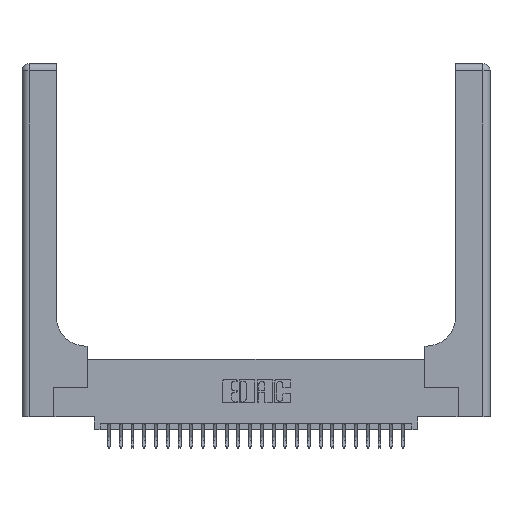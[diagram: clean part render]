
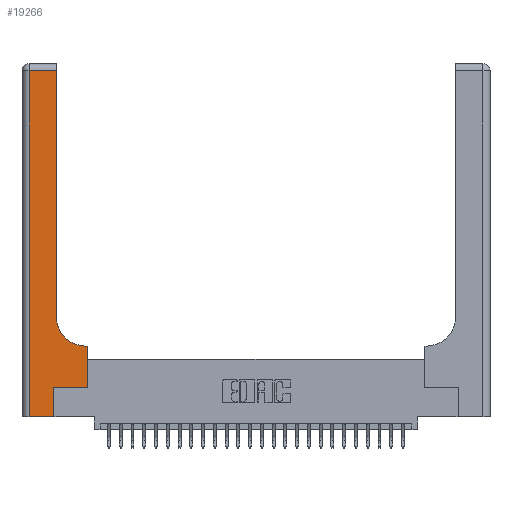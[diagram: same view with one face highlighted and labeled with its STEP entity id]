
A CAD part, top view. The second image highlights one B-rep face of the part: STEP entity #19266.
In plain terms, the highlighted planar face has unit normal (0, 0, 1).
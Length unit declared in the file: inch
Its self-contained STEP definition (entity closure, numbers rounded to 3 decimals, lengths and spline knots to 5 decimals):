
#473 = CARTESIAN_POINT ( 'NONE',  ( 0.2915, 2.94, 0.37 ) ) ;
#1381 = DIRECTION ( 'NONE',  ( 0., 1., 0. ) ) ;
#1568 = CARTESIAN_POINT ( 'NONE',  ( 0.5585, 0.25, 0.37 ) ) ;
#1997 = VERTEX_POINT ( 'NONE', #9951 ) ;
#2394 = FACE_OUTER_BOUND ( 'NONE', #5670, .T. ) ;
#3526 = ORIENTED_EDGE ( 'NONE', *, *, #18394, .T. ) ;
#3707 = CARTESIAN_POINT ( 'NONE',  ( 0.2915, 3., 0.37 ) ) ;
#3811 = DIRECTION ( 'NONE',  ( -1., 0., 0. ) ) ;
#3971 = DIRECTION ( 'NONE',  ( 0., 1., 0. ) ) ;
#4874 = DIRECTION ( 'NONE',  ( -1., 0., 0. ) ) ;
#4939 = CIRCLE ( 'NONE', #16758, 0.25 ) ;
#5670 = EDGE_LOOP ( 'NONE', ( #16331, #16443, #14378, #25839, #3526, #7637, #23231, #17557, #17245 ) ) ;
#6155 = LINE ( 'NONE', #1568, #26515 ) ;
#6334 = EDGE_CURVE ( 'NONE', #27411, #19929, #20702, .T. ) ;
#7045 = VERTEX_POINT ( 'NONE', #473 ) ;
#7300 = EDGE_CURVE ( 'NONE', #12934, #10145, #14510, .T. ) ;
#7441 = VECTOR ( 'NONE', #1381, 39.37008 ) ;
#7637 = ORIENTED_EDGE ( 'NONE', *, *, #22457, .T. ) ;
#8154 = CARTESIAN_POINT ( 'NONE',  ( 0., 2.94, 0.37 ) ) ;
#8355 = VECTOR ( 'NONE', #15981, 39.37008 ) ;
#8759 = CARTESIAN_POINT ( 'NONE',  ( 0.06, 3., 0.37 ) ) ;
#9126 = CARTESIAN_POINT ( 'NONE',  ( 0., 0., 0.37 ) ) ;
#9167 = DIRECTION ( 'NONE',  ( 0., 1., 0. ) ) ;
#9366 = CARTESIAN_POINT ( 'NONE',  ( 0.269, 0.25, 0.37 ) ) ;
#9592 = VECTOR ( 'NONE', #9167, 39.37008 ) ;
#9951 = CARTESIAN_POINT ( 'NONE',  ( 0.5585, 0.25, 0.37 ) ) ;
#10145 = VERTEX_POINT ( 'NONE', #27791 ) ;
#10206 = VERTEX_POINT ( 'NONE', #25548 ) ;
#11107 = CARTESIAN_POINT ( 'NONE',  ( 0., 3., 0.37 ) ) ;
#11243 = DIRECTION ( 'NONE',  ( 0., 0., -1. ) ) ;
#11430 = CARTESIAN_POINT ( 'NONE',  ( 0.2915, 0.6, 0.37 ) ) ;
#11555 = VECTOR ( 'NONE', #3811, 39.37008 ) ;
#12934 = VERTEX_POINT ( 'NONE', #14967 ) ;
#12981 = VERTEX_POINT ( 'NONE', #15341 ) ;
#13124 = DIRECTION ( 'NONE',  ( 0., -1., 0. ) ) ;
#13723 = CARTESIAN_POINT ( 'NONE',  ( 0.5415, 0.6, 0.37 ) ) ;
#14378 = ORIENTED_EDGE ( 'NONE', *, *, #7300, .T. ) ;
#14384 = CARTESIAN_POINT ( 'NONE',  ( 0.2915, 0.85, 0.37 ) ) ;
#14467 = EDGE_CURVE ( 'NONE', #10145, #10206, #18913, .T. ) ;
#14510 = LINE ( 'NONE', #8759, #19618 ) ;
#14879 = LINE ( 'NONE', #3707, #7441 ) ;
#14967 = CARTESIAN_POINT ( 'NONE',  ( 0.06, 2.94, 0.37 ) ) ;
#15284 = PLANE ( 'NONE',  #17898 ) ;
#15341 = CARTESIAN_POINT ( 'NONE',  ( 0.269, 0.25, 0.37 ) ) ;
#15981 = DIRECTION ( 'NONE',  ( 1., 0., 0. ) ) ;
#16331 = ORIENTED_EDGE ( 'NONE', *, *, #20767, .T. ) ;
#16443 = ORIENTED_EDGE ( 'NONE', *, *, #19646, .T. ) ;
#16758 = AXIS2_PLACEMENT_3D ( 'NONE', #26977, #11243, #26426 ) ;
#16892 = LINE ( 'NONE', #9366, #23323 ) ;
#17168 = EDGE_CURVE ( 'NONE', #19929, #25767, #4939, .T. ) ;
#17245 = ORIENTED_EDGE ( 'NONE', *, *, #17168, .T. ) ;
#17557 = ORIENTED_EDGE ( 'NONE', *, *, #6334, .T. ) ;
#17898 = AXIS2_PLACEMENT_3D ( 'NONE', #11107, #19869, #4874 ) ;
#18111 = CARTESIAN_POINT ( 'NONE',  ( 0.269, 0., 0.37 ) ) ;
#18394 = EDGE_CURVE ( 'NONE', #10206, #12981, #25899, .T. ) ;
#18913 = LINE ( 'NONE', #9126, #8355 ) ;
#19266 = ADVANCED_FACE ( 'NONE', ( #2394 ), #15284, .F. ) ;
#19618 = VECTOR ( 'NONE', #13124, 39.37008 ) ;
#19646 = EDGE_CURVE ( 'NONE', #7045, #12934, #23104, .T. ) ;
#19869 = DIRECTION ( 'NONE',  ( 0., 0., -1. ) ) ;
#19929 = VERTEX_POINT ( 'NONE', #13723 ) ;
#20702 = LINE ( 'NONE', #11430, #23734 ) ;
#20767 = EDGE_CURVE ( 'NONE', #25767, #7045, #14879, .T. ) ;
#20924 = CARTESIAN_POINT ( 'NONE',  ( 0.5585, 0.6, 0.37 ) ) ;
#22457 = EDGE_CURVE ( 'NONE', #12981, #1997, #16892, .T. ) ;
#23104 = LINE ( 'NONE', #8154, #11555 ) ;
#23231 = ORIENTED_EDGE ( 'NONE', *, *, #26873, .T. ) ;
#23323 = VECTOR ( 'NONE', #27000, 39.37008 ) ;
#23734 = VECTOR ( 'NONE', #26432, 39.37008 ) ;
#25548 = CARTESIAN_POINT ( 'NONE',  ( 0.269, 0., 0.37 ) ) ;
#25767 = VERTEX_POINT ( 'NONE', #14384 ) ;
#25839 = ORIENTED_EDGE ( 'NONE', *, *, #14467, .T. ) ;
#25899 = LINE ( 'NONE', #18111, #9592 ) ;
#26426 = DIRECTION ( 'NONE',  ( 1., 0., 0. ) ) ;
#26432 = DIRECTION ( 'NONE',  ( -1., 0., 0. ) ) ;
#26515 = VECTOR ( 'NONE', #3971, 39.37008 ) ;
#26873 = EDGE_CURVE ( 'NONE', #1997, #27411, #6155, .T. ) ;
#26977 = CARTESIAN_POINT ( 'NONE',  ( 0.5415, 0.85, 0.37 ) ) ;
#27000 = DIRECTION ( 'NONE',  ( 1., 0., 0. ) ) ;
#27411 = VERTEX_POINT ( 'NONE', #20924 ) ;
#27791 = CARTESIAN_POINT ( 'NONE',  ( 0.06, 0., 0.37 ) ) ;
